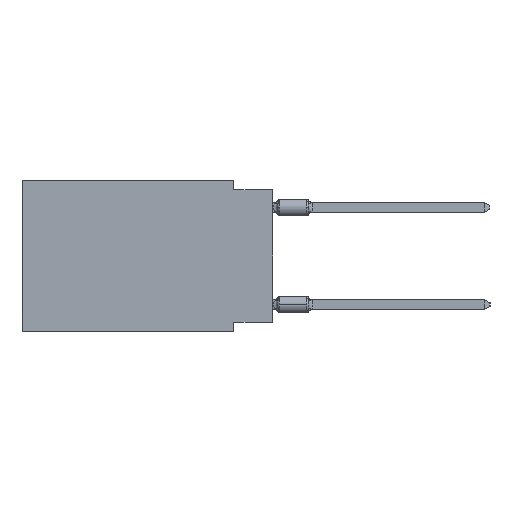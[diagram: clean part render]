
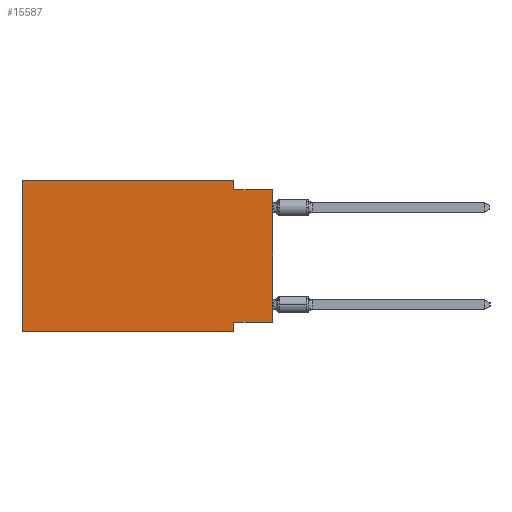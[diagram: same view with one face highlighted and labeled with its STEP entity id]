
A CAD part, left-side view. The second image highlights one B-rep face of the part: STEP entity #15587.
In plain terms, the highlighted planar face has unit normal (-1, 0, 0).
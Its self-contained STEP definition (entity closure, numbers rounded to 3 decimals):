
#1124 = LINE ( 'NONE', #5848, #5377 ) ;
#2972 = DIRECTION ( 'NONE',  ( 0., 0., -1. ) ) ;
#3249 = LINE ( 'NONE', #34511, #33622 ) ;
#3459 = VECTOR ( 'NONE', #20084, 1000. ) ;
#4355 = EDGE_CURVE ( 'NONE', #21979, #28230, #1124, .T. ) ;
#4589 = PLANE ( 'NONE',  #9913 ) ;
#4667 = EDGE_CURVE ( 'NONE', #21747, #21979, #36466, .T. ) ;
#4969 = DIRECTION ( 'NONE',  ( 0., 0., -1. ) ) ;
#5081 = EDGE_LOOP ( 'NONE', ( #35385, #7181, #23607, #25645, #25562, #24435, #13969, #11899 ) ) ;
#5182 = DIRECTION ( 'NONE',  ( 0., -1., 0. ) ) ;
#5309 = CARTESIAN_POINT ( 'NONE',  ( 0., 16.383, 0. ) ) ;
#5377 = VECTOR ( 'NONE', #12280, 1000. ) ;
#5393 = VERTEX_POINT ( 'NONE', #14629 ) ;
#5848 = CARTESIAN_POINT ( 'NONE',  ( 0., 0., -0.635 ) ) ;
#5855 = VECTOR ( 'NONE', #10498, 1000. ) ;
#6667 = EDGE_CURVE ( 'NONE', #8462, #35328, #19723, .T. ) ;
#6899 = EDGE_CURVE ( 'NONE', #5393, #16590, #14040, .T. ) ;
#7181 = ORIENTED_EDGE ( 'NONE', *, *, #4355, .F. ) ;
#7772 = CARTESIAN_POINT ( 'NONE',  ( 0., 16.383, 0. ) ) ;
#8110 = CARTESIAN_POINT ( 'NONE',  ( 0., 0., -0.635 ) ) ;
#8462 = VERTEX_POINT ( 'NONE', #35204 ) ;
#9913 = AXIS2_PLACEMENT_3D ( 'NONE', #22456, #33614, #4969 ) ;
#10498 = DIRECTION ( 'NONE',  ( 0., 0., 1. ) ) ;
#10690 = DIRECTION ( 'NONE',  ( 0., 1., 0. ) ) ;
#10964 = CARTESIAN_POINT ( 'NONE',  ( 0., 2.54, -9.906 ) ) ;
#11899 = ORIENTED_EDGE ( 'NONE', *, *, #33319, .F. ) ;
#12110 = CARTESIAN_POINT ( 'NONE',  ( 0., 2.54, -9.906 ) ) ;
#12280 = DIRECTION ( 'NONE',  ( 0., -1., 0. ) ) ;
#13294 = LINE ( 'NONE', #24830, #23637 ) ;
#13460 = VECTOR ( 'NONE', #18038, 1000. ) ;
#13969 = ORIENTED_EDGE ( 'NONE', *, *, #6667, .F. ) ;
#14040 = LINE ( 'NONE', #5309, #5855 ) ;
#14617 = EDGE_CURVE ( 'NONE', #5393, #35328, #34977, .T. ) ;
#14629 = CARTESIAN_POINT ( 'NONE',  ( 0., 16.383, -9.906 ) ) ;
#14798 = DIRECTION ( 'NONE',  ( 0., 0., 1. ) ) ;
#15587 = ADVANCED_FACE ( 'NONE', ( #30461 ), #4589, .F. ) ;
#16590 = VERTEX_POINT ( 'NONE', #20320 ) ;
#16688 = VECTOR ( 'NONE', #2972, 1000. ) ;
#18038 = DIRECTION ( 'NONE',  ( 0., -1., 0. ) ) ;
#19723 = LINE ( 'NONE', #10964, #3459 ) ;
#20084 = DIRECTION ( 'NONE',  ( 0., 0., -1. ) ) ;
#20320 = CARTESIAN_POINT ( 'NONE',  ( 0., 16.383, 0. ) ) ;
#21747 = VERTEX_POINT ( 'NONE', #29698 ) ;
#21979 = VERTEX_POINT ( 'NONE', #36568 ) ;
#22456 = CARTESIAN_POINT ( 'NONE',  ( 0., 16.383, 0. ) ) ;
#22590 = CARTESIAN_POINT ( 'NONE',  ( 0., 0., -9.271 ) ) ;
#22840 = VERTEX_POINT ( 'NONE', #22590 ) ;
#23607 = ORIENTED_EDGE ( 'NONE', *, *, #4667, .F. ) ;
#23637 = VECTOR ( 'NONE', #10690, 1000. ) ;
#24435 = ORIENTED_EDGE ( 'NONE', *, *, #14617, .T. ) ;
#24830 = CARTESIAN_POINT ( 'NONE',  ( 0., 0., -9.271 ) ) ;
#25562 = ORIENTED_EDGE ( 'NONE', *, *, #6899, .F. ) ;
#25645 = ORIENTED_EDGE ( 'NONE', *, *, #32163, .F. ) ;
#25847 = CARTESIAN_POINT ( 'NONE',  ( 0., 2.54, 0. ) ) ;
#28230 = VERTEX_POINT ( 'NONE', #8110 ) ;
#29698 = CARTESIAN_POINT ( 'NONE',  ( 0., 2.54, 0. ) ) ;
#30119 = VECTOR ( 'NONE', #5182, 1000. ) ;
#30461 = FACE_OUTER_BOUND ( 'NONE', #5081, .T. ) ;
#31066 = EDGE_CURVE ( 'NONE', #22840, #28230, #3249, .T. ) ;
#32163 = EDGE_CURVE ( 'NONE', #16590, #21747, #33274, .T. ) ;
#32189 = CARTESIAN_POINT ( 'NONE',  ( 0., 16.383, -9.906 ) ) ;
#33274 = LINE ( 'NONE', #7772, #30119 ) ;
#33319 = EDGE_CURVE ( 'NONE', #22840, #8462, #13294, .T. ) ;
#33614 = DIRECTION ( 'NONE',  ( 1., 0., 0. ) ) ;
#33622 = VECTOR ( 'NONE', #14798, 1000. ) ;
#34511 = CARTESIAN_POINT ( 'NONE',  ( 0., 0., 0. ) ) ;
#34977 = LINE ( 'NONE', #32189, #13460 ) ;
#35204 = CARTESIAN_POINT ( 'NONE',  ( 0., 2.54, -9.271 ) ) ;
#35328 = VERTEX_POINT ( 'NONE', #12110 ) ;
#35385 = ORIENTED_EDGE ( 'NONE', *, *, #31066, .T. ) ;
#36466 = LINE ( 'NONE', #25847, #16688 ) ;
#36568 = CARTESIAN_POINT ( 'NONE',  ( 0., 2.54, -0.635 ) ) ;
